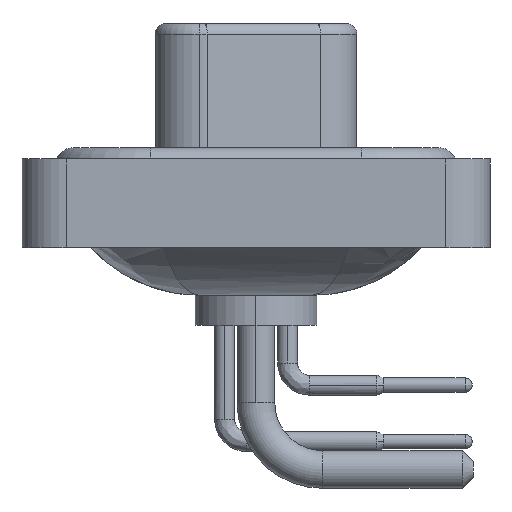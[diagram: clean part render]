
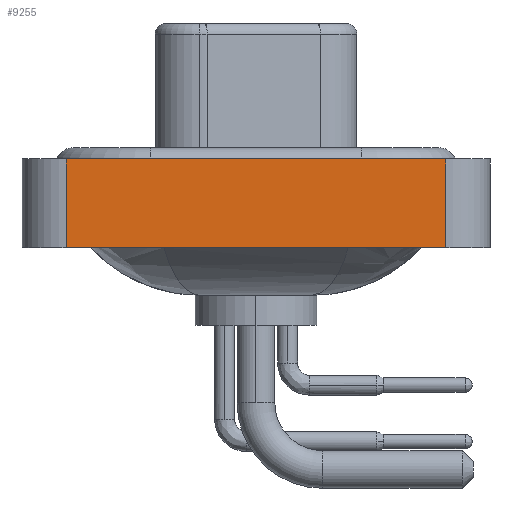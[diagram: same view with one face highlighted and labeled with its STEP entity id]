
A CAD part, left-side view. The second image highlights one B-rep face of the part: STEP entity #9255.
In plain terms, the highlighted planar face has unit normal (-1, 0, 0).
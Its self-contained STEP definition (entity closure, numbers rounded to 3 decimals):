
#529 = CARTESIAN_POINT ( 'NONE',  ( -7.35, 8.55, -3.6 ) ) ;
#836 = CARTESIAN_POINT ( 'NONE',  ( -7.35, -8.55, -3.6 ) ) ;
#1206 = LINE ( 'NONE', #836, #21866 ) ;
#1576 = EDGE_CURVE ( 'NONE', #9122, #9546, #20685, .T. ) ;
#1615 = EDGE_CURVE ( 'NONE', #13324, #2403, #19605, .T. ) ;
#2293 = CARTESIAN_POINT ( 'NONE',  ( -7.35, 8.55, 0.4 ) ) ;
#2403 = VERTEX_POINT ( 'NONE', #4161 ) ;
#4161 = CARTESIAN_POINT ( 'NONE',  ( -7.35, -8.55, 0.4 ) ) ;
#4223 = CARTESIAN_POINT ( 'NONE',  ( -7.35, -8.55, 0.4 ) ) ;
#4328 = ORIENTED_EDGE ( 'NONE', *, *, #11026, .T. ) ;
#4966 = PLANE ( 'NONE',  #6437 ) ;
#5094 = FACE_OUTER_BOUND ( 'NONE', #14869, .T. ) ;
#5202 = DIRECTION ( 'NONE',  ( 0., -1., 0. ) ) ;
#5506 = VECTOR ( 'NONE', #13480, 1000. ) ;
#6437 = AXIS2_PLACEMENT_3D ( 'NONE', #16913, #15415, #6974 ) ;
#6773 = VECTOR ( 'NONE', #22788, 1000. ) ;
#6974 = DIRECTION ( 'NONE',  ( 0., 0., 1. ) ) ;
#8469 = DIRECTION ( 'NONE',  ( 0., -1., 0. ) ) ;
#9122 = VERTEX_POINT ( 'NONE', #16510 ) ;
#9255 = ADVANCED_FACE ( 'NONE', ( #5094 ), #4966, .T. ) ;
#9546 = VERTEX_POINT ( 'NONE', #2293 ) ;
#11026 = EDGE_CURVE ( 'NONE', #9122, #13324, #1206, .T. ) ;
#11835 = EDGE_CURVE ( 'NONE', #9546, #2403, #14278, .T. ) ;
#13324 = VERTEX_POINT ( 'NONE', #15042 ) ;
#13480 = DIRECTION ( 'NONE',  ( 0., 0., 1. ) ) ;
#14278 = LINE ( 'NONE', #4223, #22948 ) ;
#14869 = EDGE_LOOP ( 'NONE', ( #15865, #24319, #25734, #4328 ) ) ;
#15042 = CARTESIAN_POINT ( 'NONE',  ( -7.35, -8.55, -3.6 ) ) ;
#15415 = DIRECTION ( 'NONE',  ( -1., 0., 0. ) ) ;
#15865 = ORIENTED_EDGE ( 'NONE', *, *, #1615, .T. ) ;
#16510 = CARTESIAN_POINT ( 'NONE',  ( -7.35, 8.55, -3.6 ) ) ;
#16913 = CARTESIAN_POINT ( 'NONE',  ( -7.35, -8.55, -3.6 ) ) ;
#17484 = CARTESIAN_POINT ( 'NONE',  ( -7.35, -8.55, -3.6 ) ) ;
#19605 = LINE ( 'NONE', #17484, #5506 ) ;
#20685 = LINE ( 'NONE', #529, #6773 ) ;
#21866 = VECTOR ( 'NONE', #5202, 1000. ) ;
#22788 = DIRECTION ( 'NONE',  ( 0., 0., 1. ) ) ;
#22948 = VECTOR ( 'NONE', #8469, 1000. ) ;
#24319 = ORIENTED_EDGE ( 'NONE', *, *, #11835, .F. ) ;
#25734 = ORIENTED_EDGE ( 'NONE', *, *, #1576, .F. ) ;
